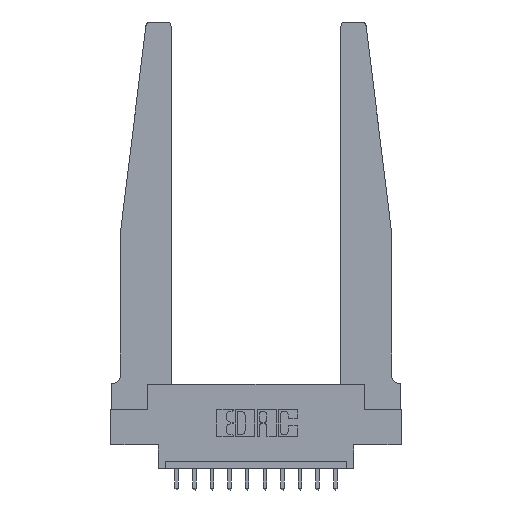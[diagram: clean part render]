
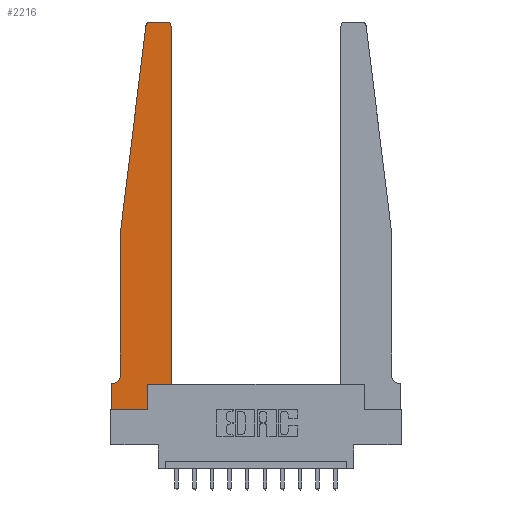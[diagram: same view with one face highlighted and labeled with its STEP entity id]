
A CAD part, top view. The second image highlights one B-rep face of the part: STEP entity #2216.
In plain terms, the highlighted planar face has unit normal (0, 0, 1).
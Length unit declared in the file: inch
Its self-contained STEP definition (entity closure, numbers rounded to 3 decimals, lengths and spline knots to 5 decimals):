
#76 = EDGE_CURVE ( 'NONE', #14037, #13010, #12052, .T. ) ;
#82 = DIRECTION ( 'NONE',  ( 1., 0., 0. ) ) ;
#172 = LINE ( 'NONE', #14777, #411 ) ;
#411 = VECTOR ( 'NONE', #12400, 39.37008 ) ;
#454 = EDGE_CURVE ( 'NONE', #11367, #3374, #15113, .T. ) ;
#526 = DIRECTION ( 'NONE',  ( 1., 0., 0. ) ) ;
#676 = CARTESIAN_POINT ( 'NONE',  ( 0., 0., 0.37 ) ) ;
#997 = CARTESIAN_POINT ( 'NONE',  ( 0.2605, 0.18, 0.37 ) ) ;
#1549 = CARTESIAN_POINT ( 'NONE',  ( 0.25, 2.75, 0.37 ) ) ;
#1981 = ORIENTED_EDGE ( 'NONE', *, *, #15735, .T. ) ;
#2029 = FACE_OUTER_BOUND ( 'NONE', #12145, .T. ) ;
#2216 = ADVANCED_FACE ( 'NONE', ( #2029 ), #5701, .T. ) ;
#2341 = DIRECTION ( 'NONE',  ( 1., 0., 0. ) ) ;
#2433 = ORIENTED_EDGE ( 'NONE', *, *, #13334, .T. ) ;
#2728 = EDGE_CURVE ( 'NONE', #10062, #13442, #6765, .T. ) ;
#2807 = DIRECTION ( 'NONE',  ( -0.122, -0.992, 0. ) ) ;
#2832 = EDGE_CURVE ( 'NONE', #11394, #8627, #3917, .T. ) ;
#2934 = ORIENTED_EDGE ( 'NONE', *, *, #454, .T. ) ;
#3186 = DIRECTION ( 'NONE',  ( 0., 1., 0. ) ) ;
#3374 = VERTEX_POINT ( 'NONE', #7212 ) ;
#3481 = VECTOR ( 'NONE', #2807, 39.37008 ) ;
#3543 = EDGE_CURVE ( 'NONE', #13123, #11367, #10281, .T. ) ;
#3607 = LINE ( 'NONE', #11027, #12371 ) ;
#3917 = CIRCLE ( 'NONE', #6248, 0.03 ) ;
#3921 = LINE ( 'NONE', #1549, #14254 ) ;
#3992 = ORIENTED_EDGE ( 'NONE', *, *, #76, .T. ) ;
#4202 = CARTESIAN_POINT ( 'NONE',  ( 0.425, 0.18, 0.37 ) ) ;
#4285 = DIRECTION ( 'NONE',  ( -1., 0., 0. ) ) ;
#4410 = DIRECTION ( 'NONE',  ( 0., -1., 0. ) ) ;
#4558 = CIRCLE ( 'NONE', #13573, 0.05 ) ;
#4710 = VECTOR ( 'NONE', #7443, 39.37008 ) ;
#4909 = EDGE_CURVE ( 'NONE', #11112, #15834, #7611, .T. ) ;
#4954 = CARTESIAN_POINT ( 'NONE',  ( 0.2605, 0., 0.37 ) ) ;
#5611 = EDGE_CURVE ( 'NONE', #13442, #13123, #172, .T. ) ;
#5648 = VECTOR ( 'NONE', #526, 39.37008 ) ;
#5701 = PLANE ( 'NONE',  #8509 ) ;
#5895 = CARTESIAN_POINT ( 'NONE',  ( 0.24675, 2.72367, 0.37 ) ) ;
#5942 = CARTESIAN_POINT ( 'NONE',  ( 0.395, 2.75, 0.37 ) ) ;
#6248 = AXIS2_PLACEMENT_3D ( 'NONE', #7148, #12077, #10802 ) ;
#6765 = LINE ( 'NONE', #676, #15690 ) ;
#6892 = DIRECTION ( 'NONE',  ( 0., 0., 1. ) ) ;
#7034 = ORIENTED_EDGE ( 'NONE', *, *, #13277, .T. ) ;
#7074 = CARTESIAN_POINT ( 'NONE',  ( 0.27653, 2.75, 0.37 ) ) ;
#7108 = ORIENTED_EDGE ( 'NONE', *, *, #8025, .T. ) ;
#7148 = CARTESIAN_POINT ( 'NONE',  ( 0.27653, 2.72, 0.37 ) ) ;
#7212 = CARTESIAN_POINT ( 'NONE',  ( 0.425, 0.18, 0.37 ) ) ;
#7414 = CARTESIAN_POINT ( 'NONE',  ( 0., 0., 0.37 ) ) ;
#7443 = DIRECTION ( 'NONE',  ( 0., -1., 0. ) ) ;
#7461 = CARTESIAN_POINT ( 'NONE',  ( 0.065, 1.25, 0.37 ) ) ;
#7496 = CARTESIAN_POINT ( 'NONE',  ( 0., 0.1875, 0.37 ) ) ;
#7611 = LINE ( 'NONE', #12524, #4710 ) ;
#7781 = CARTESIAN_POINT ( 'NONE',  ( 0.395, 2.72, 0.37 ) ) ;
#8025 = EDGE_CURVE ( 'NONE', #3374, #14037, #3607, .T. ) ;
#8120 = ORIENTED_EDGE ( 'NONE', *, *, #2832, .T. ) ;
#8509 = AXIS2_PLACEMENT_3D ( 'NONE', #9542, #6892, #2341 ) ;
#8627 = VERTEX_POINT ( 'NONE', #5895 ) ;
#8902 = DIRECTION ( 'NONE',  ( -1., 0., 0. ) ) ;
#9413 = ORIENTED_EDGE ( 'NONE', *, *, #15675, .T. ) ;
#9542 = CARTESIAN_POINT ( 'NONE',  ( 0., 0.1875, 0.37 ) ) ;
#9660 = CARTESIAN_POINT ( 'NONE',  ( 0.065, 1.25, 0.37 ) ) ;
#9968 = ORIENTED_EDGE ( 'NONE', *, *, #4909, .T. ) ;
#9979 = CARTESIAN_POINT ( 'NONE',  ( 0.015, 0.1875, 0.37 ) ) ;
#10062 = VERTEX_POINT ( 'NONE', #7496 ) ;
#10281 = LINE ( 'NONE', #10371, #14685 ) ;
#10371 = CARTESIAN_POINT ( 'NONE',  ( 0.2605, 0.18, 0.37 ) ) ;
#10750 = CARTESIAN_POINT ( 'NONE',  ( 0.015, 0.2375, 0.37 ) ) ;
#10802 = DIRECTION ( 'NONE',  ( 1., 0., 0. ) ) ;
#11027 = CARTESIAN_POINT ( 'NONE',  ( 0.425, 0.18, 0.37 ) ) ;
#11112 = VERTEX_POINT ( 'NONE', #9660 ) ;
#11367 = VERTEX_POINT ( 'NONE', #997 ) ;
#11394 = VERTEX_POINT ( 'NONE', #7074 ) ;
#12052 = CIRCLE ( 'NONE', #15731, 0.03 ) ;
#12077 = DIRECTION ( 'NONE',  ( 0., 0., 1. ) ) ;
#12145 = EDGE_LOOP ( 'NONE', ( #9413, #8120, #1981, #9968, #2433, #7034, #15794, #15285, #15792, #2934, #7108, #3992 ) ) ;
#12229 = DIRECTION ( 'NONE',  ( 0., 1., 0. ) ) ;
#12309 = DIRECTION ( 'NONE',  ( 0., 0., 1. ) ) ;
#12371 = VECTOR ( 'NONE', #12229, 39.37008 ) ;
#12400 = DIRECTION ( 'NONE',  ( 1., 0., 0. ) ) ;
#12403 = CARTESIAN_POINT ( 'NONE',  ( 0.425, 2.72, 0.37 ) ) ;
#12463 = LINE ( 'NONE', #7461, #3481 ) ;
#12524 = CARTESIAN_POINT ( 'NONE',  ( 0.065, 1.25, 0.37 ) ) ;
#12927 = DIRECTION ( 'NONE',  ( -1., 0., 0. ) ) ;
#13010 = VERTEX_POINT ( 'NONE', #5942 ) ;
#13123 = VERTEX_POINT ( 'NONE', #4954 ) ;
#13277 = EDGE_CURVE ( 'NONE', #13491, #10062, #14265, .T. ) ;
#13334 = EDGE_CURVE ( 'NONE', #15834, #13491, #4558, .T. ) ;
#13442 = VERTEX_POINT ( 'NONE', #7414 ) ;
#13491 = VERTEX_POINT ( 'NONE', #9979 ) ;
#13573 = AXIS2_PLACEMENT_3D ( 'NONE', #10750, #15587, #12927 ) ;
#13997 = CARTESIAN_POINT ( 'NONE',  ( 0.065, 0.2375, 0.37 ) ) ;
#14037 = VERTEX_POINT ( 'NONE', #12403 ) ;
#14254 = VECTOR ( 'NONE', #8902, 39.37008 ) ;
#14265 = LINE ( 'NONE', #15275, #15070 ) ;
#14685 = VECTOR ( 'NONE', #3186, 39.37008 ) ;
#14777 = CARTESIAN_POINT ( 'NONE',  ( 0., 0., 0.37 ) ) ;
#15070 = VECTOR ( 'NONE', #4285, 39.37008 ) ;
#15113 = LINE ( 'NONE', #4202, #5648 ) ;
#15275 = CARTESIAN_POINT ( 'NONE',  ( 0.065, 0.1875, 0.37 ) ) ;
#15285 = ORIENTED_EDGE ( 'NONE', *, *, #5611, .T. ) ;
#15587 = DIRECTION ( 'NONE',  ( 0., 0., -1. ) ) ;
#15675 = EDGE_CURVE ( 'NONE', #13010, #11394, #3921, .T. ) ;
#15690 = VECTOR ( 'NONE', #4410, 39.37008 ) ;
#15731 = AXIS2_PLACEMENT_3D ( 'NONE', #7781, #12309, #82 ) ;
#15735 = EDGE_CURVE ( 'NONE', #8627, #11112, #12463, .T. ) ;
#15792 = ORIENTED_EDGE ( 'NONE', *, *, #3543, .T. ) ;
#15794 = ORIENTED_EDGE ( 'NONE', *, *, #2728, .T. ) ;
#15834 = VERTEX_POINT ( 'NONE', #13997 ) ;
